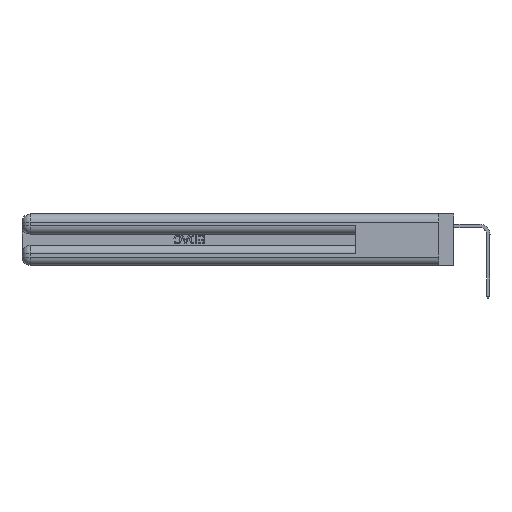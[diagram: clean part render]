
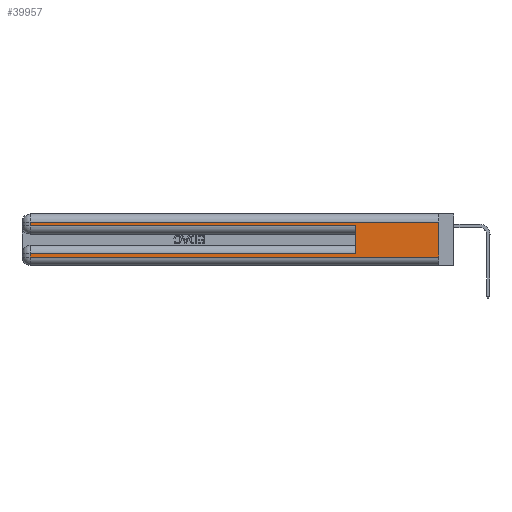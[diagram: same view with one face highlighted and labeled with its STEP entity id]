
A CAD part, left-side view. The second image highlights one B-rep face of the part: STEP entity #39957.
In plain terms, the highlighted planar face has unit normal (-1, 0, 0).
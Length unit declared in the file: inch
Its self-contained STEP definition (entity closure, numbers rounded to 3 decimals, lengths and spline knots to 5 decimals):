
#756 = ORIENTED_EDGE ( 'NONE', *, *, #25407, .T. ) ;
#1461 = CARTESIAN_POINT ( 'NONE',  ( 0., 0., 0.31 ) ) ;
#4030 = ORIENTED_EDGE ( 'NONE', *, *, #26517, .T. ) ;
#4105 = LINE ( 'NONE', #19734, #13774 ) ;
#4294 = CARTESIAN_POINT ( 'NONE',  ( 0., 2.94, 0.37 ) ) ;
#6695 = LINE ( 'NONE', #8679, #24693 ) ;
#8401 = DIRECTION ( 'NONE',  ( 0., 0., -1. ) ) ;
#8679 = CARTESIAN_POINT ( 'NONE',  ( 0., 0., 0.06 ) ) ;
#9785 = VECTOR ( 'NONE', #8401, 39.37008 ) ;
#9939 = VERTEX_POINT ( 'NONE', #11942 ) ;
#11022 = EDGE_CURVE ( 'NONE', #9939, #16840, #40677, .T. ) ;
#11322 = EDGE_CURVE ( 'NONE', #9939, #13707, #45783, .T. ) ;
#11673 = VECTOR ( 'NONE', #21944, 39.37008 ) ;
#11694 = DIRECTION ( 'NONE',  ( 0., 0., -1. ) ) ;
#11942 = CARTESIAN_POINT ( 'NONE',  ( 0., 0.6, 0.085 ) ) ;
#12435 = CARTESIAN_POINT ( 'NONE',  ( 0., 0.6, 0.145 ) ) ;
#12436 = AXIS2_PLACEMENT_3D ( 'NONE', #32135, #23896, #11694 ) ;
#13036 = ORIENTED_EDGE ( 'NONE', *, *, #15214, .F. ) ;
#13707 = VERTEX_POINT ( 'NONE', #45341 ) ;
#13774 = VECTOR ( 'NONE', #48326, 39.37008 ) ;
#14594 = DIRECTION ( 'NONE',  ( 0., 0., -1. ) ) ;
#15044 = EDGE_LOOP ( 'NONE', ( #13036, #22003, #4030, #47608, #18827, #20091, #50125, #756 ) ) ;
#15214 = EDGE_CURVE ( 'NONE', #29390, #38184, #29344, .T. ) ;
#16840 = VERTEX_POINT ( 'NONE', #48992 ) ;
#17026 = VERTEX_POINT ( 'NONE', #25580 ) ;
#18827 = ORIENTED_EDGE ( 'NONE', *, *, #11022, .F. ) ;
#19013 = DIRECTION ( 'NONE',  ( 0., 1., 0. ) ) ;
#19734 = CARTESIAN_POINT ( 'NONE',  ( 0., 2.94, 0.37 ) ) ;
#20091 = ORIENTED_EDGE ( 'NONE', *, *, #11322, .T. ) ;
#20200 = VECTOR ( 'NONE', #41055, 39.37008 ) ;
#20753 = VECTOR ( 'NONE', #42686, 39.37008 ) ;
#20911 = DIRECTION ( 'NONE',  ( 0., -1., 0. ) ) ;
#21717 = EDGE_CURVE ( 'NONE', #34868, #16840, #31657, .T. ) ;
#21944 = DIRECTION ( 'NONE',  ( 0., 1., 0. ) ) ;
#21994 = LINE ( 'NONE', #4294, #9785 ) ;
#22003 = ORIENTED_EDGE ( 'NONE', *, *, #27697, .T. ) ;
#23876 = LINE ( 'NONE', #1461, #11673 ) ;
#23896 = DIRECTION ( 'NONE',  ( 1., 0., 0. ) ) ;
#24012 = VECTOR ( 'NONE', #19013, 39.37008 ) ;
#24661 = FACE_OUTER_BOUND ( 'NONE', #15044, .T. ) ;
#24693 = VECTOR ( 'NONE', #20911, 39.37008 ) ;
#24829 = CARTESIAN_POINT ( 'NONE',  ( 0., 0., 0.06 ) ) ;
#25407 = EDGE_CURVE ( 'NONE', #28117, #38184, #6695, .T. ) ;
#25580 = CARTESIAN_POINT ( 'NONE',  ( 0., 2.94, 0.31 ) ) ;
#26517 = EDGE_CURVE ( 'NONE', #17026, #34868, #4105, .T. ) ;
#26778 = CARTESIAN_POINT ( 'NONE',  ( 0., 0., 0.37 ) ) ;
#27697 = EDGE_CURVE ( 'NONE', #29390, #17026, #23876, .T. ) ;
#28117 = VERTEX_POINT ( 'NONE', #44995 ) ;
#29344 = LINE ( 'NONE', #26778, #38888 ) ;
#29390 = VERTEX_POINT ( 'NONE', #45565 ) ;
#30352 = CARTESIAN_POINT ( 'NONE',  ( 0., 0., 0.285 ) ) ;
#31657 = LINE ( 'NONE', #30352, #20753 ) ;
#32135 = CARTESIAN_POINT ( 'NONE',  ( 0., 0., 0.37 ) ) ;
#34868 = VERTEX_POINT ( 'NONE', #35882 ) ;
#35882 = CARTESIAN_POINT ( 'NONE',  ( 0., 2.94, 0.285 ) ) ;
#36224 = PLANE ( 'NONE',  #12436 ) ;
#37062 = EDGE_CURVE ( 'NONE', #13707, #28117, #21994, .T. ) ;
#38184 = VERTEX_POINT ( 'NONE', #24829 ) ;
#38888 = VECTOR ( 'NONE', #14594, 39.37008 ) ;
#39957 = ADVANCED_FACE ( 'NONE', ( #24661 ), #36224, .F. ) ;
#40677 = LINE ( 'NONE', #12435, #20200 ) ;
#41055 = DIRECTION ( 'NONE',  ( 0., 0., 1. ) ) ;
#42686 = DIRECTION ( 'NONE',  ( 0., -1., 0. ) ) ;
#44995 = CARTESIAN_POINT ( 'NONE',  ( 0., 2.94, 0.06 ) ) ;
#45341 = CARTESIAN_POINT ( 'NONE',  ( 0., 2.94, 0.085 ) ) ;
#45565 = CARTESIAN_POINT ( 'NONE',  ( 0., 0., 0.31 ) ) ;
#45783 = LINE ( 'NONE', #46757, #24012 ) ;
#46757 = CARTESIAN_POINT ( 'NONE',  ( 0., 0., 0.085 ) ) ;
#47608 = ORIENTED_EDGE ( 'NONE', *, *, #21717, .T. ) ;
#48326 = DIRECTION ( 'NONE',  ( 0., 0., -1. ) ) ;
#48992 = CARTESIAN_POINT ( 'NONE',  ( 0., 0.6, 0.285 ) ) ;
#50125 = ORIENTED_EDGE ( 'NONE', *, *, #37062, .T. ) ;
